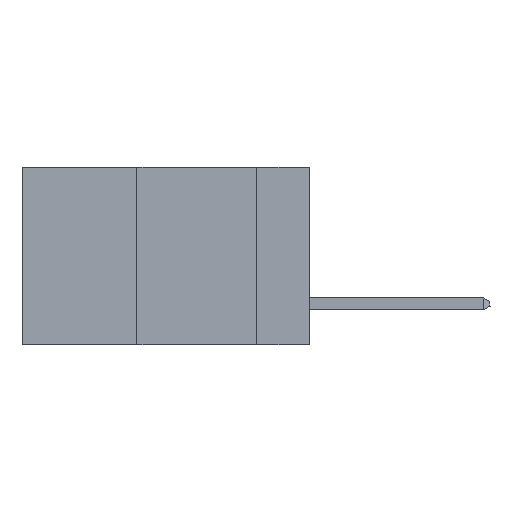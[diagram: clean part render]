
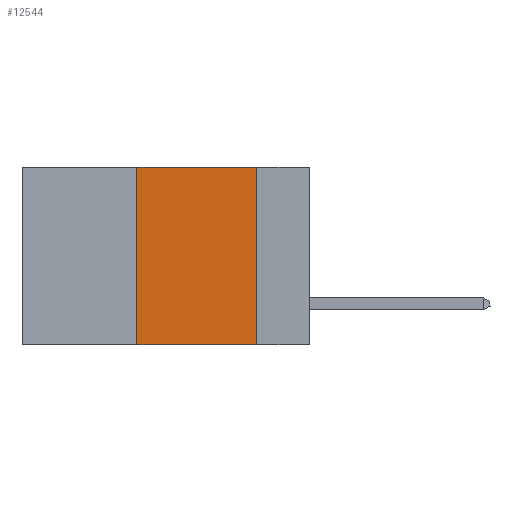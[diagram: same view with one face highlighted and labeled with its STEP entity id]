
A CAD part, left-side view. The second image highlights one B-rep face of the part: STEP entity #12544.
In plain terms, the highlighted planar face has unit normal (-1, 0, 0).
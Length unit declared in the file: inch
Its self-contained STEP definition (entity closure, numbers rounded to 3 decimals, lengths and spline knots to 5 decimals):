
#540 = VERTEX_POINT ( 'NONE', #6389 ) ;
#998 = DIRECTION ( 'NONE',  ( 0., 0., -1. ) ) ;
#2739 = VECTOR ( 'NONE', #11559, 39.37008 ) ;
#5152 = ORIENTED_EDGE ( 'NONE', *, *, #22752, .F. ) ;
#5762 = VECTOR ( 'NONE', #22552, 39.37008 ) ;
#6389 = CARTESIAN_POINT ( 'NONE',  ( 0., 0.11, -0.37 ) ) ;
#7115 = VERTEX_POINT ( 'NONE', #27227 ) ;
#8818 = EDGE_CURVE ( 'NONE', #25701, #540, #15633, .T. ) ;
#9443 = VECTOR ( 'NONE', #26095, 39.37008 ) ;
#9882 = EDGE_LOOP ( 'NONE', ( #10554, #5152, #25644, #20394 ) ) ;
#10554 = ORIENTED_EDGE ( 'NONE', *, *, #15897, .F. ) ;
#10608 = CARTESIAN_POINT ( 'NONE',  ( 0., 0.6, -0.37 ) ) ;
#10708 = AXIS2_PLACEMENT_3D ( 'NONE', #19943, #26290, #998 ) ;
#11559 = DIRECTION ( 'NONE',  ( 0., -1., 0. ) ) ;
#11627 = LINE ( 'NONE', #24630, #16234 ) ;
#11896 = VERTEX_POINT ( 'NONE', #15105 ) ;
#12118 = EDGE_CURVE ( 'NONE', #25701, #7115, #11627, .T. ) ;
#12544 = ADVANCED_FACE ( 'NONE', ( #24450 ), #15712, .F. ) ;
#15105 = CARTESIAN_POINT ( 'NONE',  ( 0., 0.11, 0. ) ) ;
#15218 = CARTESIAN_POINT ( 'NONE',  ( 0., 0.36, -0.37 ) ) ;
#15633 = LINE ( 'NONE', #10608, #2739 ) ;
#15712 = PLANE ( 'NONE',  #10708 ) ;
#15897 = EDGE_CURVE ( 'NONE', #11896, #540, #15990, .T. ) ;
#15990 = LINE ( 'NONE', #17627, #9443 ) ;
#16020 = CARTESIAN_POINT ( 'NONE',  ( 0., 0.6, 0. ) ) ;
#16234 = VECTOR ( 'NONE', #24919, 39.37008 ) ;
#17290 = LINE ( 'NONE', #16020, #5762 ) ;
#17627 = CARTESIAN_POINT ( 'NONE',  ( 0., 0.11, 0. ) ) ;
#19943 = CARTESIAN_POINT ( 'NONE',  ( 0., 0.6, 0. ) ) ;
#20394 = ORIENTED_EDGE ( 'NONE', *, *, #8818, .T. ) ;
#22552 = DIRECTION ( 'NONE',  ( 0., -1., 0. ) ) ;
#22752 = EDGE_CURVE ( 'NONE', #7115, #11896, #17290, .T. ) ;
#24450 = FACE_OUTER_BOUND ( 'NONE', #9882, .T. ) ;
#24630 = CARTESIAN_POINT ( 'NONE',  ( 0., 0.36, 0. ) ) ;
#24919 = DIRECTION ( 'NONE',  ( 0., 0., 1. ) ) ;
#25644 = ORIENTED_EDGE ( 'NONE', *, *, #12118, .F. ) ;
#25701 = VERTEX_POINT ( 'NONE', #15218 ) ;
#26095 = DIRECTION ( 'NONE',  ( 0., 0., -1. ) ) ;
#26290 = DIRECTION ( 'NONE',  ( 1., 0., 0. ) ) ;
#27227 = CARTESIAN_POINT ( 'NONE',  ( 0., 0.36, 0. ) ) ;
